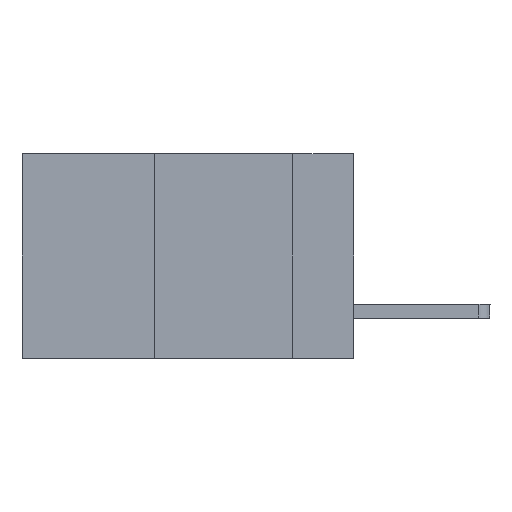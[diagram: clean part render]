
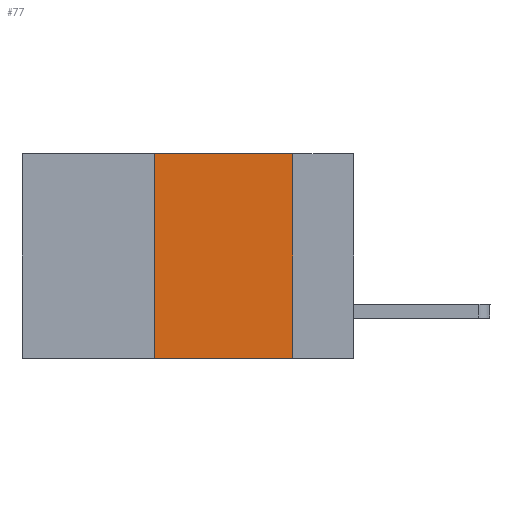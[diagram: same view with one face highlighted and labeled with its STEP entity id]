
A CAD part, left-side view. The second image highlights one B-rep face of the part: STEP entity #77.
In plain terms, the highlighted planar face has unit normal (-1, 0, 0).
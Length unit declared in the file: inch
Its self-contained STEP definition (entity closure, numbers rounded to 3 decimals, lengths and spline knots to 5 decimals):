
#77 = ADVANCED_FACE ( 'NONE', ( #9266 ), #5629, .F. ) ;
#268 = VECTOR ( 'NONE', #8227, 39.37008 ) ;
#292 = CARTESIAN_POINT ( 'NONE',  ( 0., 0.11, 0. ) ) ;
#477 = AXIS2_PLACEMENT_3D ( 'NONE', #9916, #7381, #3029 ) ;
#2174 = CARTESIAN_POINT ( 'NONE',  ( 0., 0.6, 0. ) ) ;
#2273 = CARTESIAN_POINT ( 'NONE',  ( 0., 0.6, -0.37 ) ) ;
#2287 = VERTEX_POINT ( 'NONE', #11247 ) ;
#2886 = CARTESIAN_POINT ( 'NONE',  ( 0., 0.36, 0. ) ) ;
#2962 = CARTESIAN_POINT ( 'NONE',  ( 0., 0.36, 0. ) ) ;
#3029 = DIRECTION ( 'NONE',  ( 0., 0., -1. ) ) ;
#4077 = CARTESIAN_POINT ( 'NONE',  ( 0., 0.36, -0.37 ) ) ;
#4109 = EDGE_CURVE ( 'NONE', #6258, #10221, #7027, .T. ) ;
#4227 = EDGE_CURVE ( 'NONE', #6258, #9199, #4624, .T. ) ;
#4624 = LINE ( 'NONE', #2962, #8425 ) ;
#5629 = PLANE ( 'NONE',  #477 ) ;
#6013 = LINE ( 'NONE', #2174, #8491 ) ;
#6193 = EDGE_CURVE ( 'NONE', #2287, #10221, #8915, .T. ) ;
#6258 = VERTEX_POINT ( 'NONE', #4077 ) ;
#6448 = VECTOR ( 'NONE', #8253, 39.37008 ) ;
#6916 = ORIENTED_EDGE ( 'NONE', *, *, #10699, .F. ) ;
#7027 = LINE ( 'NONE', #2273, #268 ) ;
#7381 = DIRECTION ( 'NONE',  ( 1., 0., 0. ) ) ;
#8078 = DIRECTION ( 'NONE',  ( 0., -1., 0. ) ) ;
#8227 = DIRECTION ( 'NONE',  ( 0., -1., 0. ) ) ;
#8253 = DIRECTION ( 'NONE',  ( 0., 0., -1. ) ) ;
#8425 = VECTOR ( 'NONE', #8502, 39.37008 ) ;
#8491 = VECTOR ( 'NONE', #8078, 39.37008 ) ;
#8502 = DIRECTION ( 'NONE',  ( 0., 0., 1. ) ) ;
#8915 = LINE ( 'NONE', #292, #6448 ) ;
#9034 = ORIENTED_EDGE ( 'NONE', *, *, #4109, .T. ) ;
#9199 = VERTEX_POINT ( 'NONE', #2886 ) ;
#9266 = FACE_OUTER_BOUND ( 'NONE', #9913, .T. ) ;
#9899 = ORIENTED_EDGE ( 'NONE', *, *, #6193, .F. ) ;
#9913 = EDGE_LOOP ( 'NONE', ( #9899, #6916, #10384, #9034 ) ) ;
#9916 = CARTESIAN_POINT ( 'NONE',  ( 0., 0.6, 0. ) ) ;
#10221 = VERTEX_POINT ( 'NONE', #10838 ) ;
#10384 = ORIENTED_EDGE ( 'NONE', *, *, #4227, .F. ) ;
#10699 = EDGE_CURVE ( 'NONE', #9199, #2287, #6013, .T. ) ;
#10838 = CARTESIAN_POINT ( 'NONE',  ( 0., 0.11, -0.37 ) ) ;
#11247 = CARTESIAN_POINT ( 'NONE',  ( 0., 0.11, 0. ) ) ;
